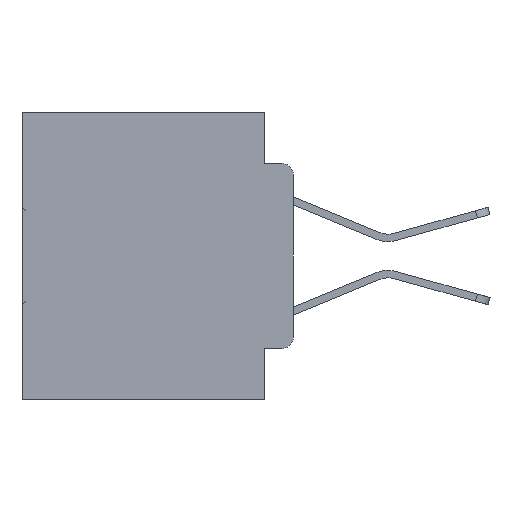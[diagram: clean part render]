
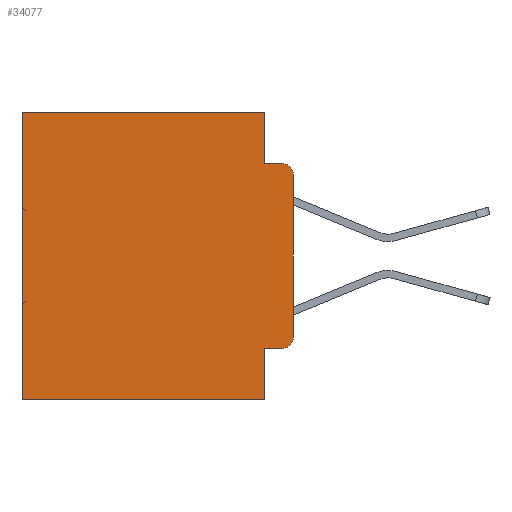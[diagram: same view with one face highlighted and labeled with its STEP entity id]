
A CAD part, left-side view. The second image highlights one B-rep face of the part: STEP entity #34077.
In plain terms, the highlighted planar face has unit normal (-1, 0, 0).
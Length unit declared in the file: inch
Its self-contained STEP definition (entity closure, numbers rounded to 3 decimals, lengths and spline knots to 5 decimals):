
#57 = LINE ( 'NONE', #9922, #26019 ) ;
#116 = DIRECTION ( 'NONE',  ( 0., 0., -1. ) ) ;
#343 = VERTEX_POINT ( 'NONE', #35658 ) ;
#454 = EDGE_CURVE ( 'NONE', #13587, #35174, #32515, .T. ) ;
#2425 = CARTESIAN_POINT ( 'NONE',  ( 0.298, 0.02, -0.3915 ) ) ;
#3249 = EDGE_CURVE ( 'NONE', #35852, #7189, #18666, .T. ) ;
#3473 = CARTESIAN_POINT ( 'NONE',  ( 0.298, 0.051, -0.4115 ) ) ;
#3562 = DIRECTION ( 'NONE',  ( 0., 0., -1. ) ) ;
#3779 = DIRECTION ( 'NONE',  ( 0., 0., -1. ) ) ;
#3928 = CARTESIAN_POINT ( 'NONE',  ( 0.298, 0.051, 0. ) ) ;
#5334 = EDGE_CURVE ( 'NONE', #10670, #6413, #31150, .T. ) ;
#6413 = VERTEX_POINT ( 'NONE', #9950 ) ;
#7189 = VERTEX_POINT ( 'NONE', #36073 ) ;
#7671 = DIRECTION ( 'NONE',  ( 0., 1., 0. ) ) ;
#8060 = DIRECTION ( 'NONE',  ( 0., 0., -1. ) ) ;
#8433 = VERTEX_POINT ( 'NONE', #36006 ) ;
#8453 = CARTESIAN_POINT ( 'NONE',  ( 0.298, 0., 0. ) ) ;
#8560 = EDGE_CURVE ( 'NONE', #13026, #343, #19917, .T. ) ;
#9313 = DIRECTION ( 'NONE',  ( 0., 0., -1. ) ) ;
#9922 = CARTESIAN_POINT ( 'NONE',  ( 0.298, 0.051, 0. ) ) ;
#9950 = CARTESIAN_POINT ( 'NONE',  ( 0.298, 0.02, -0.4115 ) ) ;
#10009 = VECTOR ( 'NONE', #29802, 39.37008 ) ;
#10670 = VERTEX_POINT ( 'NONE', #3473 ) ;
#10672 = AXIS2_PLACEMENT_3D ( 'NONE', #8453, #28160, #116 ) ;
#11014 = EDGE_CURVE ( 'NONE', #34935, #35174, #35461, .T. ) ;
#11152 = PLANE ( 'NONE',  #10672 ) ;
#11304 = ORIENTED_EDGE ( 'NONE', *, *, #5334, .T. ) ;
#12145 = CARTESIAN_POINT ( 'NONE',  ( 0.298, 0.051, 0. ) ) ;
#12458 = AXIS2_PLACEMENT_3D ( 'NONE', #2425, #24585, #33052 ) ;
#13026 = VERTEX_POINT ( 'NONE', #12145 ) ;
#13587 = VERTEX_POINT ( 'NONE', #28700 ) ;
#13875 = ORIENTED_EDGE ( 'NONE', *, *, #19013, .F. ) ;
#14036 = DIRECTION ( 'NONE',  ( 0., 1., 0. ) ) ;
#14648 = CARTESIAN_POINT ( 'NONE',  ( 0.298, 0., 0. ) ) ;
#15715 = FACE_OUTER_BOUND ( 'NONE', #32320, .T. ) ;
#15779 = VECTOR ( 'NONE', #26466, 39.37008 ) ;
#16182 = ORIENTED_EDGE ( 'NONE', *, *, #17086, .T. ) ;
#16509 = CIRCLE ( 'NONE', #12458, 0.02 ) ;
#17086 = EDGE_CURVE ( 'NONE', #343, #7189, #32391, .T. ) ;
#17287 = AXIS2_PLACEMENT_3D ( 'NONE', #36251, #27420, #8060 ) ;
#18666 = LINE ( 'NONE', #22399, #34919 ) ;
#19013 = EDGE_CURVE ( 'NONE', #10670, #35852, #23215, .T. ) ;
#19603 = ORIENTED_EDGE ( 'NONE', *, *, #36304, .F. ) ;
#19917 = LINE ( 'NONE', #28666, #31836 ) ;
#21178 = CARTESIAN_POINT ( 'NONE',  ( 0.298, 0.051, -0.4115 ) ) ;
#22399 = CARTESIAN_POINT ( 'NONE',  ( 0.298, 0., -0.5 ) ) ;
#23215 = LINE ( 'NONE', #3928, #15779 ) ;
#23327 = ORIENTED_EDGE ( 'NONE', *, *, #3249, .F. ) ;
#23392 = CARTESIAN_POINT ( 'NONE',  ( 0.298, 0.473, 0. ) ) ;
#24412 = CARTESIAN_POINT ( 'NONE',  ( 0.298, 0.051, -0.0885 ) ) ;
#24585 = DIRECTION ( 'NONE',  ( -1., 0., 0. ) ) ;
#25172 = ORIENTED_EDGE ( 'NONE', *, *, #11014, .F. ) ;
#26019 = VECTOR ( 'NONE', #3779, 39.37008 ) ;
#26466 = DIRECTION ( 'NONE',  ( 0., 0., -1. ) ) ;
#27420 = DIRECTION ( 'NONE',  ( -1., 0., 0. ) ) ;
#27977 = VECTOR ( 'NONE', #33051, 39.37008 ) ;
#28160 = DIRECTION ( 'NONE',  ( 1., 0., 0. ) ) ;
#28213 = CARTESIAN_POINT ( 'NONE',  ( 0.298, 0.02, -0.0885 ) ) ;
#28666 = CARTESIAN_POINT ( 'NONE',  ( 0.298, 0., 0. ) ) ;
#28700 = CARTESIAN_POINT ( 'NONE',  ( 0.298, 0., -0.1085 ) ) ;
#29218 = EDGE_CURVE ( 'NONE', #6413, #8433, #16509, .T. ) ;
#29579 = ORIENTED_EDGE ( 'NONE', *, *, #8560, .T. ) ;
#29594 = LINE ( 'NONE', #14648, #30483 ) ;
#29802 = DIRECTION ( 'NONE',  ( 0., -1., 0. ) ) ;
#29852 = CARTESIAN_POINT ( 'NONE',  ( 0.298, 0.051, -0.0885 ) ) ;
#30240 = EDGE_CURVE ( 'NONE', #13587, #8433, #29594, .T. ) ;
#30483 = VECTOR ( 'NONE', #9313, 39.37008 ) ;
#31069 = VECTOR ( 'NONE', #3562, 39.37008 ) ;
#31150 = LINE ( 'NONE', #21178, #10009 ) ;
#31836 = VECTOR ( 'NONE', #7671, 39.37008 ) ;
#32320 = EDGE_LOOP ( 'NONE', ( #35230, #32496, #25172, #19603, #29579, #16182, #23327, #13875, #11304, #33139 ) ) ;
#32391 = LINE ( 'NONE', #23392, #31069 ) ;
#32496 = ORIENTED_EDGE ( 'NONE', *, *, #454, .T. ) ;
#32515 = CIRCLE ( 'NONE', #17287, 0.02 ) ;
#33051 = DIRECTION ( 'NONE',  ( 0., -1., 0. ) ) ;
#33052 = DIRECTION ( 'NONE',  ( 0., 0., -1. ) ) ;
#33139 = ORIENTED_EDGE ( 'NONE', *, *, #29218, .T. ) ;
#33598 = CARTESIAN_POINT ( 'NONE',  ( 0.298, 0.051, -0.5 ) ) ;
#34077 = ADVANCED_FACE ( 'NONE', ( #15715 ), #11152, .F. ) ;
#34919 = VECTOR ( 'NONE', #14036, 39.37008 ) ;
#34935 = VERTEX_POINT ( 'NONE', #29852 ) ;
#35174 = VERTEX_POINT ( 'NONE', #28213 ) ;
#35230 = ORIENTED_EDGE ( 'NONE', *, *, #30240, .F. ) ;
#35461 = LINE ( 'NONE', #24412, #27977 ) ;
#35658 = CARTESIAN_POINT ( 'NONE',  ( 0.298, 0.473, 0. ) ) ;
#35852 = VERTEX_POINT ( 'NONE', #33598 ) ;
#36006 = CARTESIAN_POINT ( 'NONE',  ( 0.298, 0., -0.3915 ) ) ;
#36073 = CARTESIAN_POINT ( 'NONE',  ( 0.298, 0.473, -0.5 ) ) ;
#36251 = CARTESIAN_POINT ( 'NONE',  ( 0.298, 0.02, -0.1085 ) ) ;
#36304 = EDGE_CURVE ( 'NONE', #13026, #34935, #57, .T. ) ;
